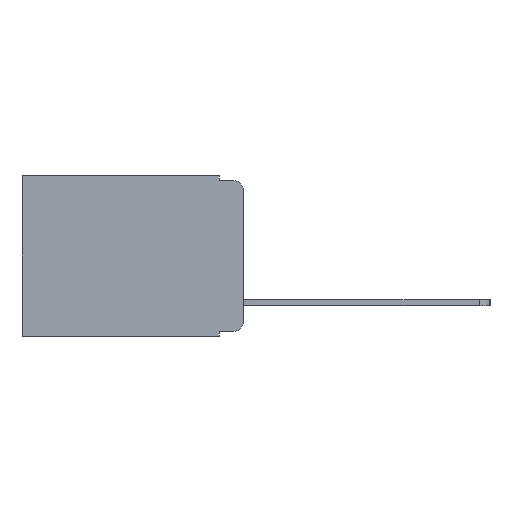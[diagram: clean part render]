
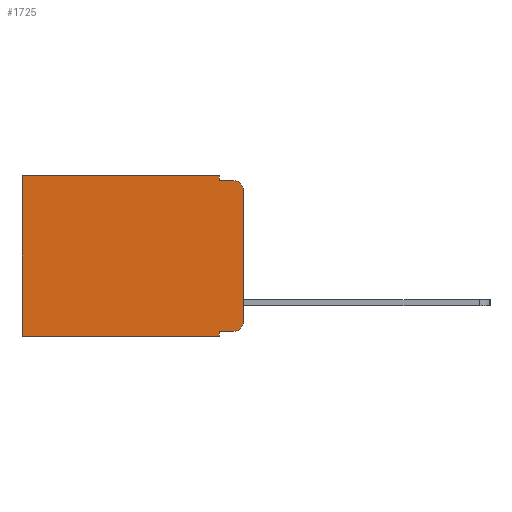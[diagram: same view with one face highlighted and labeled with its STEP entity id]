
A CAD part, left-side view. The second image highlights one B-rep face of the part: STEP entity #1725.
In plain terms, the highlighted planar face has unit normal (-1, 0, 0).
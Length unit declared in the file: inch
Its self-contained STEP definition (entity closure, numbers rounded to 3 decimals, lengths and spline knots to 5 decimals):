
#130 = LINE ( 'NONE', #8030, #494 ) ;
#306 = DIRECTION ( 'NONE',  ( -1., 0., 0. ) ) ;
#338 = DIRECTION ( 'NONE',  ( 0., 0., -1. ) ) ;
#494 = VECTOR ( 'NONE', #12309, 39.37008 ) ;
#1144 = VECTOR ( 'NONE', #4102, 39.37008 ) ;
#1572 = CARTESIAN_POINT ( 'NONE',  ( 0.298, 0.473, -0.343 ) ) ;
#1626 = ORIENTED_EDGE ( 'NONE', *, *, #6518, .T. ) ;
#1725 = ADVANCED_FACE ( 'NONE', ( #2569 ), #7851, .F. ) ;
#1919 = ORIENTED_EDGE ( 'NONE', *, *, #2764, .T. ) ;
#1954 = DIRECTION ( 'NONE',  ( 0., 0., -1. ) ) ;
#1963 = LINE ( 'NONE', #8332, #7005 ) ;
#2206 = EDGE_CURVE ( 'NONE', #5360, #12554, #7238, .T. ) ;
#2416 = ORIENTED_EDGE ( 'NONE', *, *, #10951, .F. ) ;
#2430 = ORIENTED_EDGE ( 'NONE', *, *, #4251, .F. ) ;
#2456 = AXIS2_PLACEMENT_3D ( 'NONE', #4415, #306, #338 ) ;
#2475 = ORIENTED_EDGE ( 'NONE', *, *, #2206, .T. ) ;
#2525 = VECTOR ( 'NONE', #10024, 39.37008 ) ;
#2569 = FACE_OUTER_BOUND ( 'NONE', #7026, .T. ) ;
#2642 = EDGE_CURVE ( 'NONE', #3139, #4088, #3570, .T. ) ;
#2764 = EDGE_CURVE ( 'NONE', #3139, #8979, #1963, .T. ) ;
#2847 = ORIENTED_EDGE ( 'NONE', *, *, #5870, .T. ) ;
#2949 = VERTEX_POINT ( 'NONE', #8000 ) ;
#3009 = VERTEX_POINT ( 'NONE', #3050 ) ;
#3050 = CARTESIAN_POINT ( 'NONE',  ( 0.298, 0.051, -0.343 ) ) ;
#3096 = ORIENTED_EDGE ( 'NONE', *, *, #6955, .F. ) ;
#3105 = ORIENTED_EDGE ( 'NONE', *, *, #2642, .F. ) ;
#3139 = VERTEX_POINT ( 'NONE', #12451 ) ;
#3154 = EDGE_CURVE ( 'NONE', #12503, #12509, #130, .T. ) ;
#3170 = ORIENTED_EDGE ( 'NONE', *, *, #3154, .T. ) ;
#3188 = ORIENTED_EDGE ( 'NONE', *, *, #10574, .F. ) ;
#3190 = CARTESIAN_POINT ( 'NONE',  ( 0.298, 0.051, 0. ) ) ;
#3470 = LINE ( 'NONE', #7716, #5820 ) ;
#3570 = LINE ( 'NONE', #8364, #1144 ) ;
#3643 = CARTESIAN_POINT ( 'NONE',  ( 0.298, 0.02, -0.01 ) ) ;
#4088 = VERTEX_POINT ( 'NONE', #4758 ) ;
#4102 = DIRECTION ( 'NONE',  ( 0., 0., -1. ) ) ;
#4218 = CARTESIAN_POINT ( 'NONE',  ( 0.298, 0., 0. ) ) ;
#4251 = EDGE_CURVE ( 'NONE', #5360, #2949, #12735, .T. ) ;
#4316 = AXIS2_PLACEMENT_3D ( 'NONE', #4218, #12446, #8616 ) ;
#4388 = LINE ( 'NONE', #11398, #9274 ) ;
#4403 = VECTOR ( 'NONE', #1954, 39.37008 ) ;
#4415 = CARTESIAN_POINT ( 'NONE',  ( 0.298, 0.02, -0.03 ) ) ;
#4587 = CIRCLE ( 'NONE', #11667, 0.02 ) ;
#4758 = CARTESIAN_POINT ( 'NONE',  ( 0.298, 0.051, -0.01 ) ) ;
#5360 = VERTEX_POINT ( 'NONE', #8990 ) ;
#5585 = CARTESIAN_POINT ( 'NONE',  ( 0.298, 0.02, -0.333 ) ) ;
#5818 = VERTEX_POINT ( 'NONE', #1572 ) ;
#5820 = VECTOR ( 'NONE', #12423, 39.37008 ) ;
#5870 = EDGE_CURVE ( 'NONE', #12509, #2949, #4587, .T. ) ;
#5979 = CARTESIAN_POINT ( 'NONE',  ( 0.298, 0.473, 0. ) ) ;
#6518 = EDGE_CURVE ( 'NONE', #8979, #5818, #7940, .T. ) ;
#6955 = EDGE_CURVE ( 'NONE', #3009, #5818, #4388, .T. ) ;
#7005 = VECTOR ( 'NONE', #9975, 39.37008 ) ;
#7026 = EDGE_LOOP ( 'NONE', ( #2430, #2475, #2416, #3105, #1919, #1626, #3096, #3188, #3170, #2847 ) ) ;
#7222 = DIRECTION ( 'NONE',  ( 0., 0., -1. ) ) ;
#7238 = CIRCLE ( 'NONE', #2456, 0.02 ) ;
#7331 = CARTESIAN_POINT ( 'NONE',  ( 0.298, 0., 0. ) ) ;
#7716 = CARTESIAN_POINT ( 'NONE',  ( 0.298, 0.051, -0.01 ) ) ;
#7718 = VECTOR ( 'NONE', #7222, 39.37008 ) ;
#7719 = DIRECTION ( 'NONE',  ( 0., 1., 0. ) ) ;
#7851 = PLANE ( 'NONE',  #4316 ) ;
#7940 = LINE ( 'NONE', #5979, #4403 ) ;
#8000 = CARTESIAN_POINT ( 'NONE',  ( 0.298, 0., -0.313 ) ) ;
#8030 = CARTESIAN_POINT ( 'NONE',  ( 0.298, 0.051, -0.333 ) ) ;
#8332 = CARTESIAN_POINT ( 'NONE',  ( 0.298, 0., 0. ) ) ;
#8364 = CARTESIAN_POINT ( 'NONE',  ( 0.298, 0.051, 0. ) ) ;
#8411 = DIRECTION ( 'NONE',  ( 0., 0., -1. ) ) ;
#8465 = DIRECTION ( 'NONE',  ( -1., 0., 0. ) ) ;
#8477 = CARTESIAN_POINT ( 'NONE',  ( 0.298, 0.02, -0.313 ) ) ;
#8616 = DIRECTION ( 'NONE',  ( 0., 0., -1. ) ) ;
#8979 = VERTEX_POINT ( 'NONE', #10545 ) ;
#8990 = CARTESIAN_POINT ( 'NONE',  ( 0.298, 0., -0.03 ) ) ;
#9274 = VECTOR ( 'NONE', #7719, 39.37008 ) ;
#9428 = CARTESIAN_POINT ( 'NONE',  ( 0.298, 0.051, -0.333 ) ) ;
#9975 = DIRECTION ( 'NONE',  ( 0., 1., 0. ) ) ;
#10024 = DIRECTION ( 'NONE',  ( 0., 0., -1. ) ) ;
#10321 = LINE ( 'NONE', #3190, #2525 ) ;
#10545 = CARTESIAN_POINT ( 'NONE',  ( 0.298, 0.473, 0. ) ) ;
#10574 = EDGE_CURVE ( 'NONE', #12503, #3009, #10321, .T. ) ;
#10951 = EDGE_CURVE ( 'NONE', #4088, #12554, #3470, .T. ) ;
#11398 = CARTESIAN_POINT ( 'NONE',  ( 0.298, 0., -0.343 ) ) ;
#11667 = AXIS2_PLACEMENT_3D ( 'NONE', #8477, #8465, #8411 ) ;
#12309 = DIRECTION ( 'NONE',  ( 0., -1., 0. ) ) ;
#12423 = DIRECTION ( 'NONE',  ( 0., -1., 0. ) ) ;
#12446 = DIRECTION ( 'NONE',  ( 1., 0., 0. ) ) ;
#12451 = CARTESIAN_POINT ( 'NONE',  ( 0.298, 0.051, 0. ) ) ;
#12503 = VERTEX_POINT ( 'NONE', #9428 ) ;
#12509 = VERTEX_POINT ( 'NONE', #5585 ) ;
#12554 = VERTEX_POINT ( 'NONE', #3643 ) ;
#12735 = LINE ( 'NONE', #7331, #7718 ) ;
